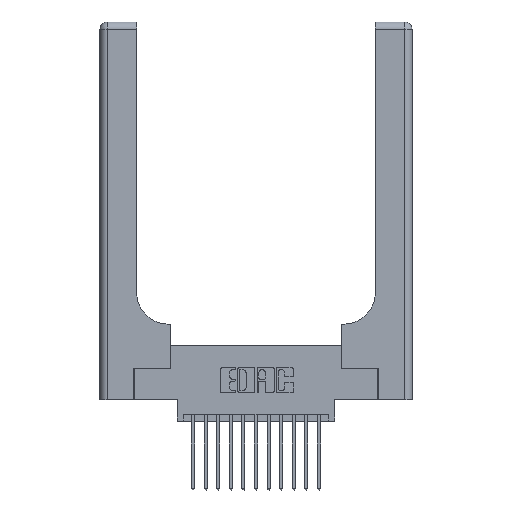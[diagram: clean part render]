
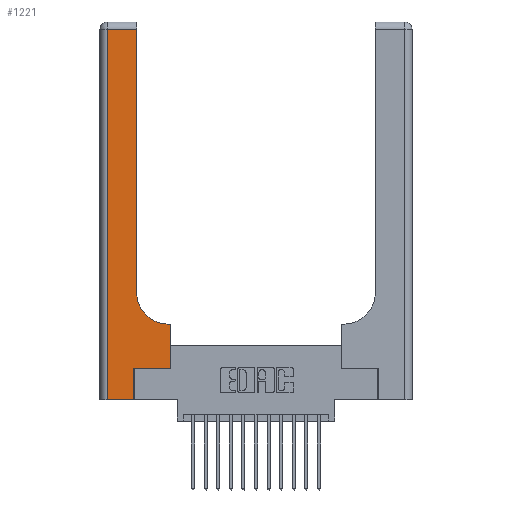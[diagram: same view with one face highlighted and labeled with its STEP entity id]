
A CAD part, top view. The second image highlights one B-rep face of the part: STEP entity #1221.
In plain terms, the highlighted planar face has unit normal (0, 0, 1).
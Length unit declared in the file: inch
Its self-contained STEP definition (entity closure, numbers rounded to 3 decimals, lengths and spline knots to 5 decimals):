
#19 = FACE_OUTER_BOUND ( 'NONE', #9803, .T. ) ;
#193 = EDGE_CURVE ( 'NONE', #12054, #14886, #13990, .T. ) ;
#220 = EDGE_CURVE ( 'NONE', #14886, #17445, #6607, .T. ) ;
#415 = CARTESIAN_POINT ( 'NONE',  ( 0.269, 0., 0.37 ) ) ;
#728 = CARTESIAN_POINT ( 'NONE',  ( 0.2915, 2.94, 0.37 ) ) ;
#945 = CARTESIAN_POINT ( 'NONE',  ( 0.5585, 0.6, 0.37 ) ) ;
#974 = ORIENTED_EDGE ( 'NONE', *, *, #13288, .T. ) ;
#989 = EDGE_CURVE ( 'NONE', #17445, #8604, #18000, .T. ) ;
#1221 = ADVANCED_FACE ( 'NONE', ( #19 ), #3364, .F. ) ;
#1676 = CARTESIAN_POINT ( 'NONE',  ( 0., 3., 0.37 ) ) ;
#1748 = VECTOR ( 'NONE', #5277, 39.37008 ) ;
#1891 = DIRECTION ( 'NONE',  ( 0., 1., 0. ) ) ;
#2206 = CARTESIAN_POINT ( 'NONE',  ( 0., 2.94, 0.37 ) ) ;
#2380 = CARTESIAN_POINT ( 'NONE',  ( 0.5415, 0.6, 0.37 ) ) ;
#2650 = CARTESIAN_POINT ( 'NONE',  ( 0.06, 0., 0.37 ) ) ;
#2681 = CARTESIAN_POINT ( 'NONE',  ( 0.5585, 0.25, 0.37 ) ) ;
#2732 = CARTESIAN_POINT ( 'NONE',  ( 0.2915, 0.85, 0.37 ) ) ;
#2961 = DIRECTION ( 'NONE',  ( -1., 0., 0. ) ) ;
#3034 = DIRECTION ( 'NONE',  ( 0., 0., -1. ) ) ;
#3069 = DIRECTION ( 'NONE',  ( 0., 0., -1. ) ) ;
#3136 = EDGE_CURVE ( 'NONE', #6820, #4590, #14931, .T. ) ;
#3364 = PLANE ( 'NONE',  #12883 ) ;
#3402 = VERTEX_POINT ( 'NONE', #2681 ) ;
#3665 = VERTEX_POINT ( 'NONE', #4670 ) ;
#4590 = VERTEX_POINT ( 'NONE', #2650 ) ;
#4670 = CARTESIAN_POINT ( 'NONE',  ( 0.269, 0., 0.37 ) ) ;
#5277 = DIRECTION ( 'NONE',  ( 1., 0., 0. ) ) ;
#5453 = ORIENTED_EDGE ( 'NONE', *, *, #3136, .T. ) ;
#5671 = VECTOR ( 'NONE', #1891, 39.37008 ) ;
#5851 = LINE ( 'NONE', #2206, #16464 ) ;
#6607 = CIRCLE ( 'NONE', #16414, 0.25 ) ;
#6820 = VERTEX_POINT ( 'NONE', #9168 ) ;
#6896 = DIRECTION ( 'NONE',  ( 0., 1., 0. ) ) ;
#7011 = VECTOR ( 'NONE', #9456, 39.37008 ) ;
#7250 = ORIENTED_EDGE ( 'NONE', *, *, #8835, .T. ) ;
#7950 = VECTOR ( 'NONE', #15222, 39.37008 ) ;
#8324 = VERTEX_POINT ( 'NONE', #10017 ) ;
#8604 = VERTEX_POINT ( 'NONE', #728 ) ;
#8835 = EDGE_CURVE ( 'NONE', #8604, #6820, #5851, .T. ) ;
#9168 = CARTESIAN_POINT ( 'NONE',  ( 0.06, 2.94, 0.37 ) ) ;
#9382 = CARTESIAN_POINT ( 'NONE',  ( 0.2915, 3., 0.37 ) ) ;
#9456 = DIRECTION ( 'NONE',  ( 0., 1., 0. ) ) ;
#9803 = EDGE_LOOP ( 'NONE', ( #16258, #7250, #5453, #10899, #13080, #974, #12008, #15879, #9846 ) ) ;
#9846 = ORIENTED_EDGE ( 'NONE', *, *, #220, .T. ) ;
#9906 = VECTOR ( 'NONE', #6896, 39.37008 ) ;
#10017 = CARTESIAN_POINT ( 'NONE',  ( 0.269, 0.25, 0.37 ) ) ;
#10329 = LINE ( 'NONE', #13806, #9906 ) ;
#10899 = ORIENTED_EDGE ( 'NONE', *, *, #17990, .T. ) ;
#10917 = CARTESIAN_POINT ( 'NONE',  ( 0.5415, 0.85, 0.37 ) ) ;
#11258 = VECTOR ( 'NONE', #12595, 39.37008 ) ;
#11419 = CARTESIAN_POINT ( 'NONE',  ( 0.2915, 0.6, 0.37 ) ) ;
#11606 = LINE ( 'NONE', #13869, #7950 ) ;
#11646 = LINE ( 'NONE', #14988, #1748 ) ;
#11726 = DIRECTION ( 'NONE',  ( 1., 0., 0. ) ) ;
#11801 = DIRECTION ( 'NONE',  ( -1., 0., 0. ) ) ;
#11913 = DIRECTION ( 'NONE',  ( -1., 0., 0. ) ) ;
#12008 = ORIENTED_EDGE ( 'NONE', *, *, #18070, .T. ) ;
#12054 = VERTEX_POINT ( 'NONE', #945 ) ;
#12595 = DIRECTION ( 'NONE',  ( 0., -1., 0. ) ) ;
#12644 = LINE ( 'NONE', #415, #5671 ) ;
#12678 = CARTESIAN_POINT ( 'NONE',  ( 0.06, 3., 0.37 ) ) ;
#12883 = AXIS2_PLACEMENT_3D ( 'NONE', #1676, #3069, #2961 ) ;
#13080 = ORIENTED_EDGE ( 'NONE', *, *, #14645, .T. ) ;
#13288 = EDGE_CURVE ( 'NONE', #8324, #3402, #11606, .T. ) ;
#13549 = VECTOR ( 'NONE', #11801, 39.37008 ) ;
#13806 = CARTESIAN_POINT ( 'NONE',  ( 0.5585, 0.25, 0.37 ) ) ;
#13869 = CARTESIAN_POINT ( 'NONE',  ( 0.269, 0.25, 0.37 ) ) ;
#13990 = LINE ( 'NONE', #11419, #13549 ) ;
#14645 = EDGE_CURVE ( 'NONE', #3665, #8324, #12644, .T. ) ;
#14886 = VERTEX_POINT ( 'NONE', #2380 ) ;
#14931 = LINE ( 'NONE', #12678, #11258 ) ;
#14988 = CARTESIAN_POINT ( 'NONE',  ( 0., 0., 0.37 ) ) ;
#15222 = DIRECTION ( 'NONE',  ( 1., 0., 0. ) ) ;
#15879 = ORIENTED_EDGE ( 'NONE', *, *, #193, .T. ) ;
#16258 = ORIENTED_EDGE ( 'NONE', *, *, #989, .T. ) ;
#16414 = AXIS2_PLACEMENT_3D ( 'NONE', #10917, #3034, #11726 ) ;
#16464 = VECTOR ( 'NONE', #11913, 39.37008 ) ;
#17445 = VERTEX_POINT ( 'NONE', #2732 ) ;
#17990 = EDGE_CURVE ( 'NONE', #4590, #3665, #11646, .T. ) ;
#18000 = LINE ( 'NONE', #9382, #7011 ) ;
#18070 = EDGE_CURVE ( 'NONE', #3402, #12054, #10329, .T. ) ;
